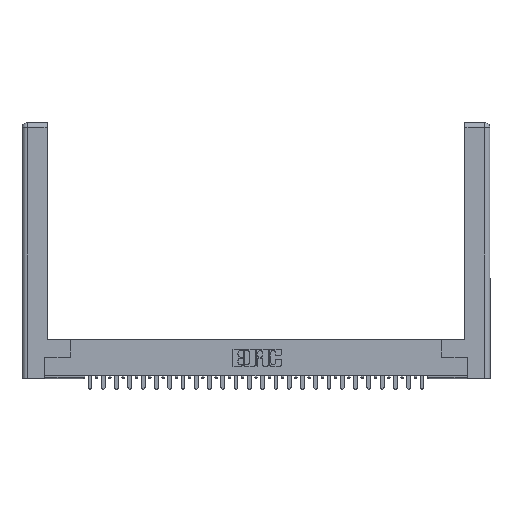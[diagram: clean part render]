
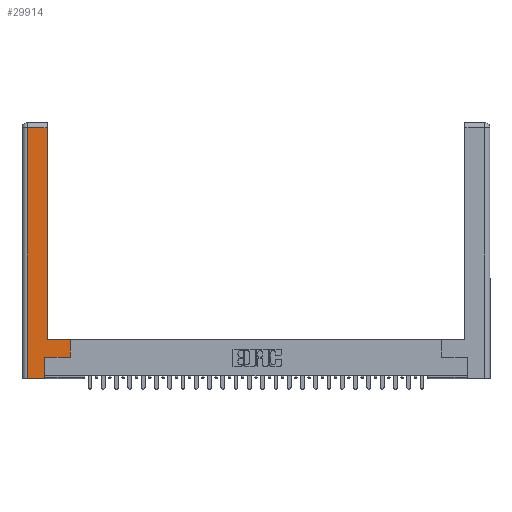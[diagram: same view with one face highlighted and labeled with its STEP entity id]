
A CAD part, top view. The second image highlights one B-rep face of the part: STEP entity #29914.
In plain terms, the highlighted planar face has unit normal (0, 0, 1).
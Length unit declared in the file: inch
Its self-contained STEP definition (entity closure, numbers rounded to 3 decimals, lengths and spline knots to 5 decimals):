
#275 = ORIENTED_EDGE ( 'NONE', *, *, #18249, .T. ) ;
#1776 = DIRECTION ( 'NONE',  ( -1., 0., 0. ) ) ;
#1899 = EDGE_CURVE ( 'NONE', #14815, #5486, #19067, .T. ) ;
#2017 = ORIENTED_EDGE ( 'NONE', *, *, #22238, .T. ) ;
#2788 = CARTESIAN_POINT ( 'NONE',  ( 0.0615, 0., 0. ) ) ;
#5019 = CARTESIAN_POINT ( 'NONE',  ( 0.265, 0., 0. ) ) ;
#5303 = VERTEX_POINT ( 'NONE', #7968 ) ;
#5320 = DIRECTION ( 'NONE',  ( 0., -1., 0. ) ) ;
#5486 = VERTEX_POINT ( 'NONE', #16361 ) ;
#6123 = LINE ( 'NONE', #15795, #11589 ) ;
#7454 = CARTESIAN_POINT ( 'NONE',  ( 0.565, 0.245, 0. ) ) ;
#7740 = DIRECTION ( 'NONE',  ( 0., 1., 0. ) ) ;
#7968 = CARTESIAN_POINT ( 'NONE',  ( 0.265, 0.245, 0. ) ) ;
#8257 = EDGE_CURVE ( 'NONE', #15917, #26539, #6123, .T. ) ;
#8881 = DIRECTION ( 'NONE',  ( 0., 0., -1. ) ) ;
#8907 = CARTESIAN_POINT ( 'NONE',  ( 0.565, 0.45, 0. ) ) ;
#9304 = ORIENTED_EDGE ( 'NONE', *, *, #28289, .T. ) ;
#9669 = AXIS2_PLACEMENT_3D ( 'NONE', #24466, #8881, #1776 ) ;
#10011 = VECTOR ( 'NONE', #17284, 39.37008 ) ;
#10599 = ORIENTED_EDGE ( 'NONE', *, *, #19266, .T. ) ;
#10686 = FACE_OUTER_BOUND ( 'NONE', #18185, .T. ) ;
#10908 = ORIENTED_EDGE ( 'NONE', *, *, #8257, .T. ) ;
#11303 = CARTESIAN_POINT ( 'NONE',  ( 0.265, 0., 0. ) ) ;
#11589 = VECTOR ( 'NONE', #31141, 39.37008 ) ;
#13345 = ORIENTED_EDGE ( 'NONE', *, *, #1899, .T. ) ;
#13892 = EDGE_CURVE ( 'NONE', #18902, #15917, #29328, .T. ) ;
#14815 = VERTEX_POINT ( 'NONE', #31167 ) ;
#15173 = LINE ( 'NONE', #21229, #32160 ) ;
#15795 = CARTESIAN_POINT ( 'NONE',  ( 0.295, 3., 0. ) ) ;
#15917 = VERTEX_POINT ( 'NONE', #28534 ) ;
#16126 = PLANE ( 'NONE',  #9669 ) ;
#16361 = CARTESIAN_POINT ( 'NONE',  ( 0.0615, 0., 0. ) ) ;
#16401 = CARTESIAN_POINT ( 'NONE',  ( 0.295, 2.94, 0. ) ) ;
#17284 = DIRECTION ( 'NONE',  ( 1., 0., 0. ) ) ;
#18185 = EDGE_LOOP ( 'NONE', ( #10908, #275, #13345, #9304, #2017, #10599, #22934, #20637 ) ) ;
#18249 = EDGE_CURVE ( 'NONE', #26539, #14815, #15173, .T. ) ;
#18587 = EDGE_CURVE ( 'NONE', #20369, #18902, #19505, .T. ) ;
#18902 = VERTEX_POINT ( 'NONE', #8907 ) ;
#18919 = DIRECTION ( 'NONE',  ( 0., 1., 0. ) ) ;
#19067 = LINE ( 'NONE', #2788, #26987 ) ;
#19266 = EDGE_CURVE ( 'NONE', #5303, #20369, #30104, .T. ) ;
#19505 = LINE ( 'NONE', #20597, #23082 ) ;
#20369 = VERTEX_POINT ( 'NONE', #21035 ) ;
#20543 = VECTOR ( 'NONE', #18919, 39.37008 ) ;
#20597 = CARTESIAN_POINT ( 'NONE',  ( 0.565, 0.45, 0. ) ) ;
#20637 = ORIENTED_EDGE ( 'NONE', *, *, #13892, .T. ) ;
#21035 = CARTESIAN_POINT ( 'NONE',  ( 0.565, 0.245, 0. ) ) ;
#21188 = VERTEX_POINT ( 'NONE', #11303 ) ;
#21229 = CARTESIAN_POINT ( 'NONE',  ( 0.0615, 2.94, 0. ) ) ;
#22238 = EDGE_CURVE ( 'NONE', #21188, #5303, #25699, .T. ) ;
#22934 = ORIENTED_EDGE ( 'NONE', *, *, #18587, .T. ) ;
#23029 = VECTOR ( 'NONE', #25095, 39.37008 ) ;
#23082 = VECTOR ( 'NONE', #7740, 39.37008 ) ;
#23432 = VECTOR ( 'NONE', #27940, 39.37008 ) ;
#24466 = CARTESIAN_POINT ( 'NONE',  ( 0., 0., 0. ) ) ;
#25095 = DIRECTION ( 'NONE',  ( -1., 0., 0. ) ) ;
#25699 = LINE ( 'NONE', #26227, #20543 ) ;
#26227 = CARTESIAN_POINT ( 'NONE',  ( 0.265, 0.245, 0. ) ) ;
#26531 = DIRECTION ( 'NONE',  ( -1., 0., 0. ) ) ;
#26539 = VERTEX_POINT ( 'NONE', #16401 ) ;
#26987 = VECTOR ( 'NONE', #5320, 39.37008 ) ;
#27001 = LINE ( 'NONE', #5019, #10011 ) ;
#27940 = DIRECTION ( 'NONE',  ( 1., 0., 0. ) ) ;
#28289 = EDGE_CURVE ( 'NONE', #5486, #21188, #27001, .T. ) ;
#28534 = CARTESIAN_POINT ( 'NONE',  ( 0.295, 0.45, 0. ) ) ;
#29328 = LINE ( 'NONE', #30025, #23029 ) ;
#29914 = ADVANCED_FACE ( 'NONE', ( #10686 ), #16126, .F. ) ;
#30025 = CARTESIAN_POINT ( 'NONE',  ( 0.295, 0.45, 0. ) ) ;
#30104 = LINE ( 'NONE', #7454, #23432 ) ;
#31141 = DIRECTION ( 'NONE',  ( 0., 1., 0. ) ) ;
#31167 = CARTESIAN_POINT ( 'NONE',  ( 0.0615, 2.94, 0. ) ) ;
#32160 = VECTOR ( 'NONE', #26531, 39.37008 ) ;
